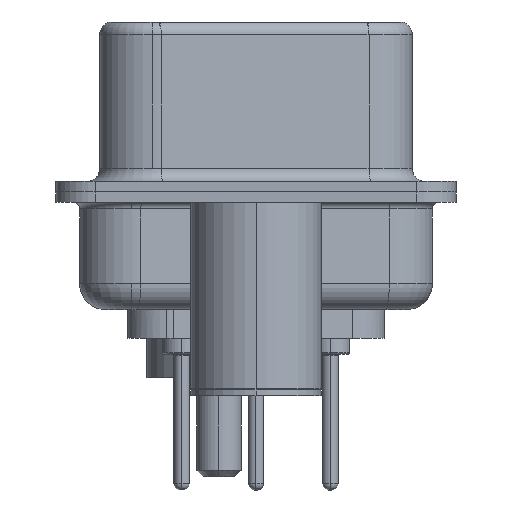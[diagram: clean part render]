
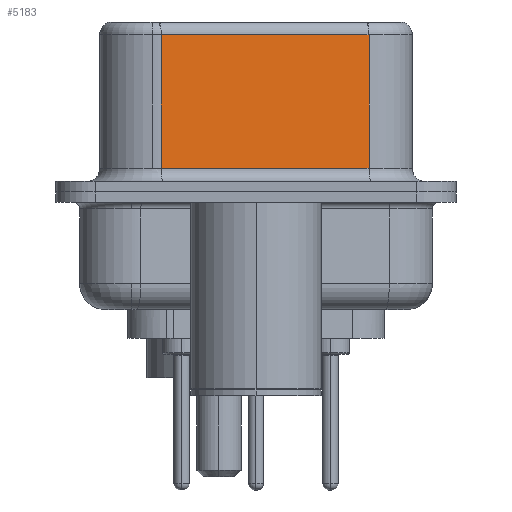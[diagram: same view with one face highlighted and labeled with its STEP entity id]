
A CAD part, left-side view. The second image highlights one B-rep face of the part: STEP entity #5183.
In plain terms, the highlighted planar face has unit normal (-0.985, -0.174, 0).
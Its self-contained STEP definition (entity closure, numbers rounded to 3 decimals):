
#2374 = ORIENTED_EDGE ( 'NONE', *, *, #27438, .T. ) ;
#2491 = VECTOR ( 'NONE', #10296, 1000. ) ;
#4057 = DIRECTION ( 'NONE',  ( 0., 0., -1. ) ) ;
#4656 = AXIS2_PLACEMENT_3D ( 'NONE', #31698, #18809, #18701 ) ;
#5183 = ADVANCED_FACE ( 'NONE', ( #28048 ), #18489, .F. ) ;
#5288 = VERTEX_POINT ( 'NONE', #8536 ) ;
#6365 = ORIENTED_EDGE ( 'NONE', *, *, #11147, .F. ) ;
#8536 = CARTESIAN_POINT ( 'NONE',  ( 3.73, 3.628, 6.02 ) ) ;
#8768 = LINE ( 'NONE', #26675, #21386 ) ;
#10296 = DIRECTION ( 'NONE',  ( -0.174, 0.985, 0. ) ) ;
#11147 = EDGE_CURVE ( 'NONE', #25435, #23902, #8768, .T. ) ;
#12465 = DIRECTION ( 'NONE',  ( 0.174, -0.985, 0. ) ) ;
#13285 = EDGE_CURVE ( 'NONE', #15783, #23902, #20124, .T. ) ;
#13396 = VECTOR ( 'NONE', #12465, 1000. ) ;
#15783 = VERTEX_POINT ( 'NONE', #29750 ) ;
#15847 = EDGE_LOOP ( 'NONE', ( #6365, #2374, #22844, #16157 ) ) ;
#16157 = ORIENTED_EDGE ( 'NONE', *, *, #13285, .T. ) ;
#17421 = LINE ( 'NONE', #17910, #2491 ) ;
#17910 = CARTESIAN_POINT ( 'NONE',  ( 5.132, -4.322, 6.02 ) ) ;
#18019 = CARTESIAN_POINT ( 'NONE',  ( 5.132, -4.322, 0.9 ) ) ;
#18489 = PLANE ( 'NONE',  #4656 ) ;
#18701 = DIRECTION ( 'NONE',  ( -0.174, 0.985, 0. ) ) ;
#18809 = DIRECTION ( 'NONE',  ( 0.985, 0.174, 0. ) ) ;
#19208 = DIRECTION ( 'NONE',  ( 0., 0., -1. ) ) ;
#20124 = LINE ( 'NONE', #30000, #13396 ) ;
#21386 = VECTOR ( 'NONE', #19208, 1000. ) ;
#21427 = CARTESIAN_POINT ( 'NONE',  ( 3.73, 3.628, 6.52 ) ) ;
#22844 = ORIENTED_EDGE ( 'NONE', *, *, #29951, .T. ) ;
#23902 = VERTEX_POINT ( 'NONE', #18019 ) ;
#25201 = LINE ( 'NONE', #21427, #30303 ) ;
#25435 = VERTEX_POINT ( 'NONE', #28950 ) ;
#26675 = CARTESIAN_POINT ( 'NONE',  ( 5.132, -4.322, 6.52 ) ) ;
#27438 = EDGE_CURVE ( 'NONE', #25435, #5288, #17421, .T. ) ;
#28048 = FACE_OUTER_BOUND ( 'NONE', #15847, .T. ) ;
#28950 = CARTESIAN_POINT ( 'NONE',  ( 5.132, -4.322, 6.02 ) ) ;
#29750 = CARTESIAN_POINT ( 'NONE',  ( 3.73, 3.628, 0.9 ) ) ;
#29951 = EDGE_CURVE ( 'NONE', #5288, #15783, #25201, .T. ) ;
#30000 = CARTESIAN_POINT ( 'NONE',  ( 5.132, -4.322, 0.9 ) ) ;
#30303 = VECTOR ( 'NONE', #4057, 1000. ) ;
#31698 = CARTESIAN_POINT ( 'NONE',  ( 5.132, -4.322, 6.52 ) ) ;
